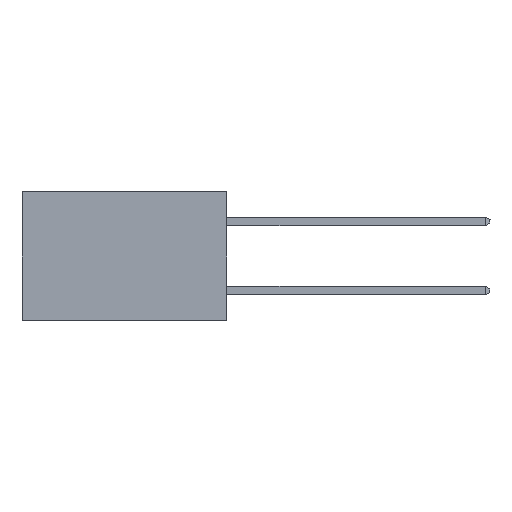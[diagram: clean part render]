
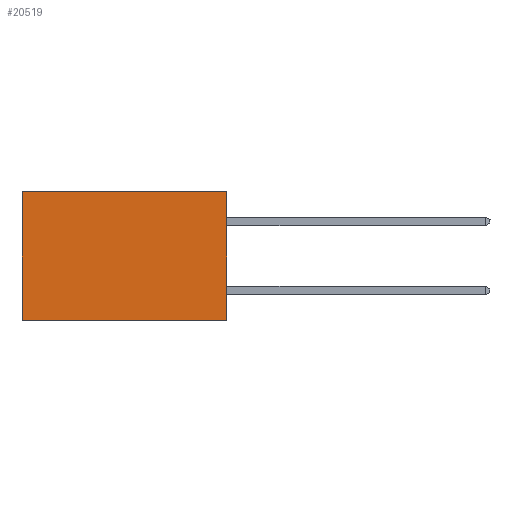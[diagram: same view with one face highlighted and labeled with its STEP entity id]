
A CAD part, left-side view. The second image highlights one B-rep face of the part: STEP entity #20519.
In plain terms, the highlighted planar face has unit normal (-1, 0, 0).
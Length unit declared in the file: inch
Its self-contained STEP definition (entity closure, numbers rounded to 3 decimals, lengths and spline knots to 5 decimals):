
#53 = FACE_OUTER_BOUND ( 'NONE', #7038, .T. ) ;
#2042 = VERTEX_POINT ( 'NONE', #20162 ) ;
#3383 = EDGE_CURVE ( 'NONE', #3654, #21944, #28879, .T. ) ;
#3654 = VERTEX_POINT ( 'NONE', #21247 ) ;
#4006 = VECTOR ( 'NONE', #6823, 39.37008 ) ;
#4436 = LINE ( 'NONE', #6169, #16558 ) ;
#4677 = DIRECTION ( 'NONE',  ( 0., 1., 0. ) ) ;
#4813 = CARTESIAN_POINT ( 'NONE',  ( 0.277, 0., 0. ) ) ;
#6169 = CARTESIAN_POINT ( 'NONE',  ( 0.277, 0., -0.37 ) ) ;
#6823 = DIRECTION ( 'NONE',  ( 0., 0., -1. ) ) ;
#7038 = EDGE_LOOP ( 'NONE', ( #7678, #14570, #28282, #17509 ) ) ;
#7152 = EDGE_CURVE ( 'NONE', #3654, #15456, #10733, .T. ) ;
#7678 = ORIENTED_EDGE ( 'NONE', *, *, #19169, .T. ) ;
#8636 = DIRECTION ( 'NONE',  ( 0., 1., 0. ) ) ;
#9098 = DIRECTION ( 'NONE',  ( 0., 0., -1. ) ) ;
#9387 = CARTESIAN_POINT ( 'NONE',  ( 0.277, 0.59, -0.37 ) ) ;
#9831 = VECTOR ( 'NONE', #17392, 39.37008 ) ;
#10733 = LINE ( 'NONE', #4813, #28997 ) ;
#14379 = AXIS2_PLACEMENT_3D ( 'NONE', #18694, #23497, #9098 ) ;
#14570 = ORIENTED_EDGE ( 'NONE', *, *, #30943, .F. ) ;
#15456 = VERTEX_POINT ( 'NONE', #18416 ) ;
#16278 = PLANE ( 'NONE',  #14379 ) ;
#16558 = VECTOR ( 'NONE', #8636, 39.37008 ) ;
#16864 = LINE ( 'NONE', #9387, #4006 ) ;
#17392 = DIRECTION ( 'NONE',  ( 0., 0., -1. ) ) ;
#17509 = ORIENTED_EDGE ( 'NONE', *, *, #7152, .T. ) ;
#18416 = CARTESIAN_POINT ( 'NONE',  ( 0.277, 0.59, 0. ) ) ;
#18694 = CARTESIAN_POINT ( 'NONE',  ( 0.277, 0., -0.37 ) ) ;
#19169 = EDGE_CURVE ( 'NONE', #15456, #2042, #16864, .T. ) ;
#20162 = CARTESIAN_POINT ( 'NONE',  ( 0.277, 0.59, -0.37 ) ) ;
#20519 = ADVANCED_FACE ( 'NONE', ( #53 ), #16278, .F. ) ;
#20968 = CARTESIAN_POINT ( 'NONE',  ( 0.277, 0., -0.37 ) ) ;
#21247 = CARTESIAN_POINT ( 'NONE',  ( 0.277, 0., 0. ) ) ;
#21944 = VERTEX_POINT ( 'NONE', #25051 ) ;
#23497 = DIRECTION ( 'NONE',  ( 1., 0., 0. ) ) ;
#25051 = CARTESIAN_POINT ( 'NONE',  ( 0.277, 0., -0.37 ) ) ;
#28282 = ORIENTED_EDGE ( 'NONE', *, *, #3383, .F. ) ;
#28879 = LINE ( 'NONE', #20968, #9831 ) ;
#28997 = VECTOR ( 'NONE', #4677, 39.37008 ) ;
#30943 = EDGE_CURVE ( 'NONE', #21944, #2042, #4436, .T. ) ;
